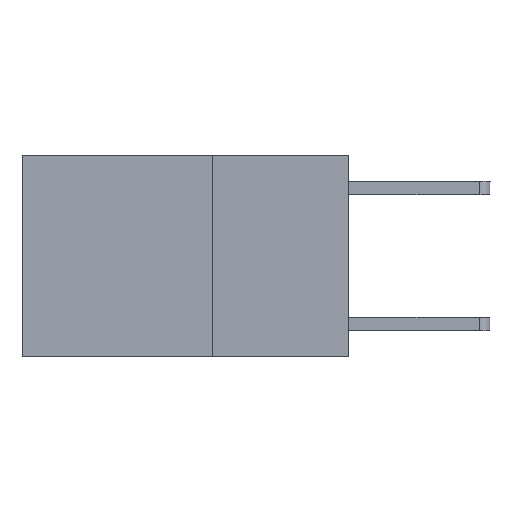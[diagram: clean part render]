
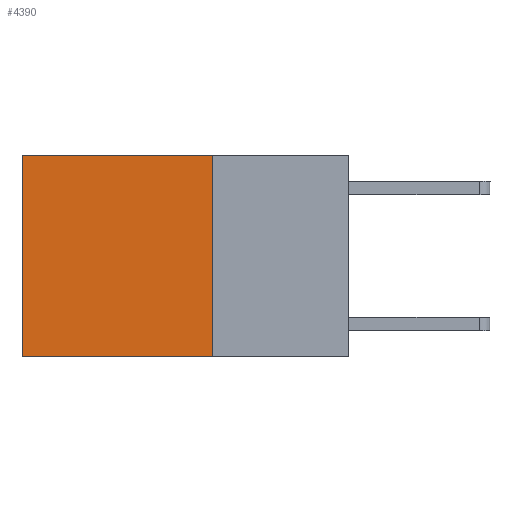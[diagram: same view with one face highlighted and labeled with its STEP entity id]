
A CAD part, left-side view. The second image highlights one B-rep face of the part: STEP entity #4390.
In plain terms, the highlighted planar face has unit normal (-1, 0, 0).
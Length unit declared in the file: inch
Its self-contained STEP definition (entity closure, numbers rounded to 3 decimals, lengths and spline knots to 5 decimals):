
#333 = EDGE_CURVE ( 'NONE', #1476, #7106, #6607, .T. ) ;
#580 = FACE_OUTER_BOUND ( 'NONE', #1706, .T. ) ;
#837 = CARTESIAN_POINT ( 'NONE',  ( 0.2625, 0.25, -0.37 ) ) ;
#1215 = CARTESIAN_POINT ( 'NONE',  ( 0.2625, 0.25, 0. ) ) ;
#1444 = CARTESIAN_POINT ( 'NONE',  ( 0.2625, 0.6, -0.37 ) ) ;
#1476 = VERTEX_POINT ( 'NONE', #5895 ) ;
#1706 = EDGE_LOOP ( 'NONE', ( #5356, #4781, #5965, #6431 ) ) ;
#2340 = VERTEX_POINT ( 'NONE', #2429 ) ;
#2429 = CARTESIAN_POINT ( 'NONE',  ( 0.2625, 0.25, -0.37 ) ) ;
#2683 = VECTOR ( 'NONE', #3203, 39.37008 ) ;
#2879 = DIRECTION ( 'NONE',  ( 1., 0., 0. ) ) ;
#3203 = DIRECTION ( 'NONE',  ( 0., 1., 0. ) ) ;
#3497 = DIRECTION ( 'NONE',  ( 0., 0., -1. ) ) ;
#3510 = EDGE_CURVE ( 'NONE', #5905, #2340, #5868, .T. ) ;
#3543 = CARTESIAN_POINT ( 'NONE',  ( 0.2625, 0.25, 0. ) ) ;
#3811 = DIRECTION ( 'NONE',  ( 0., 0., -1. ) ) ;
#4390 = ADVANCED_FACE ( 'NONE', ( #580 ), #9360, .F. ) ;
#4781 = ORIENTED_EDGE ( 'NONE', *, *, #5346, .F. ) ;
#5224 = VECTOR ( 'NONE', #8842, 39.37008 ) ;
#5246 = LINE ( 'NONE', #837, #5224 ) ;
#5346 = EDGE_CURVE ( 'NONE', #2340, #7106, #5246, .T. ) ;
#5356 = ORIENTED_EDGE ( 'NONE', *, *, #333, .T. ) ;
#5383 = EDGE_CURVE ( 'NONE', #5905, #1476, #6658, .T. ) ;
#5389 = VECTOR ( 'NONE', #7094, 39.37008 ) ;
#5830 = AXIS2_PLACEMENT_3D ( 'NONE', #3543, #2879, #3497 ) ;
#5868 = LINE ( 'NONE', #8040, #5389 ) ;
#5895 = CARTESIAN_POINT ( 'NONE',  ( 0.2625, 0.6, 0. ) ) ;
#5905 = VERTEX_POINT ( 'NONE', #1215 ) ;
#5965 = ORIENTED_EDGE ( 'NONE', *, *, #3510, .F. ) ;
#6431 = ORIENTED_EDGE ( 'NONE', *, *, #5383, .T. ) ;
#6607 = LINE ( 'NONE', #8792, #7330 ) ;
#6658 = LINE ( 'NONE', #8123, #2683 ) ;
#7094 = DIRECTION ( 'NONE',  ( 0., 0., -1. ) ) ;
#7106 = VERTEX_POINT ( 'NONE', #1444 ) ;
#7330 = VECTOR ( 'NONE', #3811, 39.37008 ) ;
#8040 = CARTESIAN_POINT ( 'NONE',  ( 0.2625, 0.25, 0. ) ) ;
#8123 = CARTESIAN_POINT ( 'NONE',  ( 0.2625, 0.25, 0. ) ) ;
#8792 = CARTESIAN_POINT ( 'NONE',  ( 0.2625, 0.6, 0. ) ) ;
#8842 = DIRECTION ( 'NONE',  ( 0., 1., 0. ) ) ;
#9360 = PLANE ( 'NONE',  #5830 ) ;
